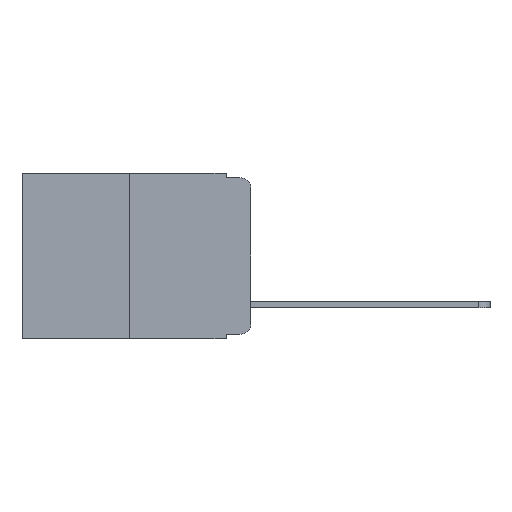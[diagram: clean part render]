
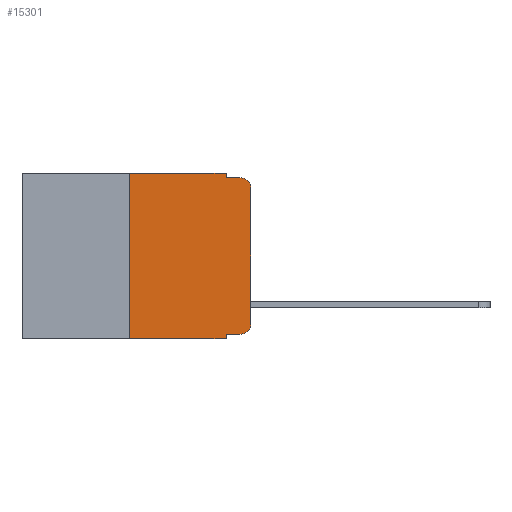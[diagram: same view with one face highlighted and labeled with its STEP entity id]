
A CAD part, left-side view. The second image highlights one B-rep face of the part: STEP entity #15301.
In plain terms, the highlighted planar face has unit normal (-1, 0, 0).
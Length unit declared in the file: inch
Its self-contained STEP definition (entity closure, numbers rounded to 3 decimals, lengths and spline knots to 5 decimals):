
#210 = CARTESIAN_POINT ( 'NONE',  ( 0., 0.02, -0.03 ) ) ;
#894 = DIRECTION ( 'NONE',  ( 0., 0., 1. ) ) ;
#952 = DIRECTION ( 'NONE',  ( 1., 0., 0. ) ) ;
#990 = LINE ( 'NONE', #7154, #7489 ) ;
#1122 = EDGE_CURVE ( 'NONE', #3758, #18824, #990, .T. ) ;
#1132 = CARTESIAN_POINT ( 'NONE',  ( 0., 0.25, 0. ) ) ;
#1166 = CARTESIAN_POINT ( 'NONE',  ( 0., 0.473, -0.343 ) ) ;
#2178 = EDGE_CURVE ( 'NONE', #12137, #8130, #18607, .T. ) ;
#2707 = VECTOR ( 'NONE', #894, 39.37008 ) ;
#3309 = ORIENTED_EDGE ( 'NONE', *, *, #12077, .T. ) ;
#3680 = EDGE_CURVE ( 'NONE', #6392, #15034, #8498, .T. ) ;
#3758 = VERTEX_POINT ( 'NONE', #8070 ) ;
#3959 = DIRECTION ( 'NONE',  ( 0., 0., -1. ) ) ;
#4044 = LINE ( 'NONE', #16558, #2707 ) ;
#4820 = CARTESIAN_POINT ( 'NONE',  ( 0., 0., 0. ) ) ;
#4997 = VECTOR ( 'NONE', #6854, 39.37008 ) ;
#5498 = VECTOR ( 'NONE', #3959, 39.37008 ) ;
#5533 = LINE ( 'NONE', #16429, #11869 ) ;
#6392 = VERTEX_POINT ( 'NONE', #20925 ) ;
#6854 = DIRECTION ( 'NONE',  ( 0., -1., 0. ) ) ;
#6863 = ORIENTED_EDGE ( 'NONE', *, *, #7012, .F. ) ;
#7012 = EDGE_CURVE ( 'NONE', #17373, #3758, #5533, .T. ) ;
#7154 = CARTESIAN_POINT ( 'NONE',  ( 0., 0.051, -0.01 ) ) ;
#7173 = CARTESIAN_POINT ( 'NONE',  ( 0., 0.051, 0. ) ) ;
#7283 = DIRECTION ( 'NONE',  ( 0., -1., 0. ) ) ;
#7406 = CARTESIAN_POINT ( 'NONE',  ( 0., 0.051, 0. ) ) ;
#7449 = LINE ( 'NONE', #4820, #13507 ) ;
#7489 = VECTOR ( 'NONE', #19320, 39.37008 ) ;
#7500 = EDGE_CURVE ( 'NONE', #10662, #12867, #7449, .T. ) ;
#7854 = CARTESIAN_POINT ( 'NONE',  ( 0., 0.473, 0. ) ) ;
#8070 = CARTESIAN_POINT ( 'NONE',  ( 0., 0.051, -0.01 ) ) ;
#8130 = VERTEX_POINT ( 'NONE', #13713 ) ;
#8249 = FACE_OUTER_BOUND ( 'NONE', #13497, .T. ) ;
#8498 = LINE ( 'NONE', #1166, #18516 ) ;
#8522 = CARTESIAN_POINT ( 'NONE',  ( 0., 0., -0.03 ) ) ;
#8632 = ORIENTED_EDGE ( 'NONE', *, *, #1122, .F. ) ;
#9003 = CARTESIAN_POINT ( 'NONE',  ( 0., 0.051, -0.333 ) ) ;
#9077 = DIRECTION ( 'NONE',  ( -1., 0., 0. ) ) ;
#9509 = DIRECTION ( 'NONE',  ( 0., 0., -1. ) ) ;
#10228 = CARTESIAN_POINT ( 'NONE',  ( 0., 0.051, -0.333 ) ) ;
#10271 = ORIENTED_EDGE ( 'NONE', *, *, #15147, .F. ) ;
#10513 = AXIS2_PLACEMENT_3D ( 'NONE', #11705, #20083, #21813 ) ;
#10662 = VERTEX_POINT ( 'NONE', #20072 ) ;
#11126 = CIRCLE ( 'NONE', #13799, 0.02 ) ;
#11128 = ORIENTED_EDGE ( 'NONE', *, *, #11277, .F. ) ;
#11277 = EDGE_CURVE ( 'NONE', #18732, #17373, #19238, .T. ) ;
#11705 = CARTESIAN_POINT ( 'NONE',  ( 0., 0.02, -0.313 ) ) ;
#11773 = AXIS2_PLACEMENT_3D ( 'NONE', #7854, #952, #13016 ) ;
#11869 = VECTOR ( 'NONE', #9509, 39.37008 ) ;
#12077 = EDGE_CURVE ( 'NONE', #12867, #18824, #11126, .T. ) ;
#12137 = VERTEX_POINT ( 'NONE', #9003 ) ;
#12531 = CARTESIAN_POINT ( 'NONE',  ( 0., 0.473, 0. ) ) ;
#12631 = DIRECTION ( 'NONE',  ( 0., 0., -1. ) ) ;
#12771 = VECTOR ( 'NONE', #7283, 39.37008 ) ;
#12867 = VERTEX_POINT ( 'NONE', #8522 ) ;
#13016 = DIRECTION ( 'NONE',  ( 0., 0., -1. ) ) ;
#13375 = DIRECTION ( 'NONE',  ( 0., -1., 0. ) ) ;
#13497 = EDGE_LOOP ( 'NONE', ( #14671, #3309, #8632, #6863, #11128, #18423, #21703, #10271, #20154, #13602 ) ) ;
#13507 = VECTOR ( 'NONE', #17011, 39.37008 ) ;
#13602 = ORIENTED_EDGE ( 'NONE', *, *, #20670, .T. ) ;
#13713 = CARTESIAN_POINT ( 'NONE',  ( 0., 0.02, -0.333 ) ) ;
#13799 = AXIS2_PLACEMENT_3D ( 'NONE', #210, #9077, #12631 ) ;
#14671 = ORIENTED_EDGE ( 'NONE', *, *, #7500, .T. ) ;
#15034 = VERTEX_POINT ( 'NONE', #19417 ) ;
#15147 = EDGE_CURVE ( 'NONE', #12137, #15034, #19918, .T. ) ;
#15301 = ADVANCED_FACE ( 'NONE', ( #8249 ), #21802, .F. ) ;
#16429 = CARTESIAN_POINT ( 'NONE',  ( 0., 0.051, 0. ) ) ;
#16558 = CARTESIAN_POINT ( 'NONE',  ( 0., 0.25, 0. ) ) ;
#16914 = EDGE_CURVE ( 'NONE', #6392, #18732, #4044, .T. ) ;
#17011 = DIRECTION ( 'NONE',  ( 0., 0., 1. ) ) ;
#17373 = VERTEX_POINT ( 'NONE', #7173 ) ;
#17979 = CIRCLE ( 'NONE', #10513, 0.02 ) ;
#18423 = ORIENTED_EDGE ( 'NONE', *, *, #16914, .F. ) ;
#18516 = VECTOR ( 'NONE', #13375, 39.37008 ) ;
#18607 = LINE ( 'NONE', #10228, #4997 ) ;
#18732 = VERTEX_POINT ( 'NONE', #1132 ) ;
#18824 = VERTEX_POINT ( 'NONE', #21994 ) ;
#19238 = LINE ( 'NONE', #12531, #12771 ) ;
#19320 = DIRECTION ( 'NONE',  ( 0., -1., 0. ) ) ;
#19417 = CARTESIAN_POINT ( 'NONE',  ( 0., 0.051, -0.343 ) ) ;
#19918 = LINE ( 'NONE', #7406, #5498 ) ;
#20072 = CARTESIAN_POINT ( 'NONE',  ( 0., 0., -0.313 ) ) ;
#20083 = DIRECTION ( 'NONE',  ( -1., 0., 0. ) ) ;
#20154 = ORIENTED_EDGE ( 'NONE', *, *, #2178, .T. ) ;
#20670 = EDGE_CURVE ( 'NONE', #8130, #10662, #17979, .T. ) ;
#20925 = CARTESIAN_POINT ( 'NONE',  ( 0., 0.25, -0.343 ) ) ;
#21703 = ORIENTED_EDGE ( 'NONE', *, *, #3680, .T. ) ;
#21802 = PLANE ( 'NONE',  #11773 ) ;
#21813 = DIRECTION ( 'NONE',  ( 0., 0., -1. ) ) ;
#21994 = CARTESIAN_POINT ( 'NONE',  ( 0., 0.02, -0.01 ) ) ;
